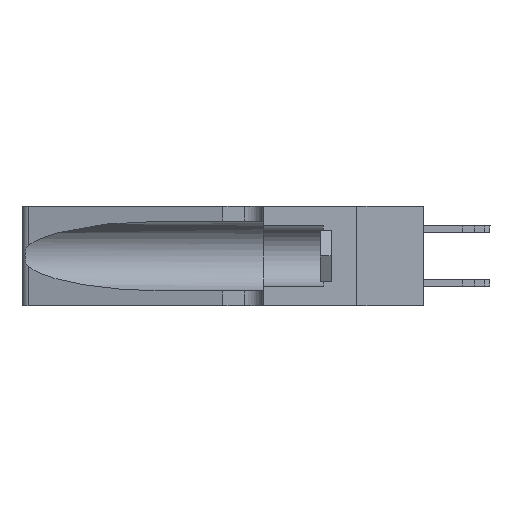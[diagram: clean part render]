
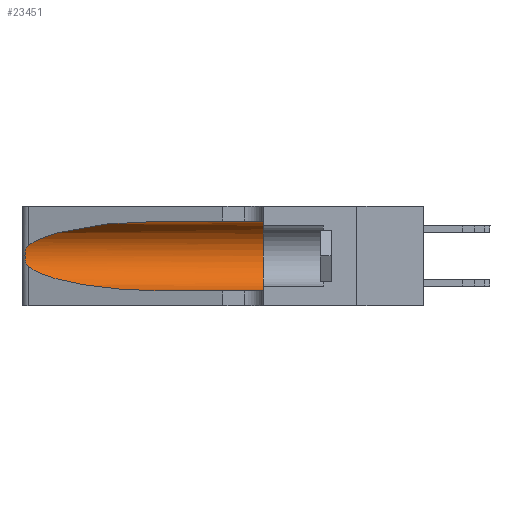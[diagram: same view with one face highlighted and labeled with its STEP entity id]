
A CAD part, left-side view. The second image highlights one B-rep face of the part: STEP entity #23451.
In plain terms, the highlighted cylindrical face has radius 3.308 mm (diameter 6.617 mm), a partial arc.
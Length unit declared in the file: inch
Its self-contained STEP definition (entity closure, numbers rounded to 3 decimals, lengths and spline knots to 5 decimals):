
#1413 = ORIENTED_EDGE ( 'NONE', *, *, #24359, .F. ) ;
#1736 = CARTESIAN_POINT ( 'NONE',  ( 0.26018, 1.23835, 0.19895 ) ) ;
#1756 = CARTESIAN_POINT ( 'NONE',  ( 0.1305, 0.35, 0.31525 ) ) ;
#2377 = CARTESIAN_POINT ( 'NONE',  ( 0.25639, 1.23184, 0.21858 ) ) ;
#2514 = CARTESIAN_POINT ( 'NONE',  ( 0.1305, 0.35, 0.05475 ) ) ;
#2838 =( BOUNDED_CURVE ( )  B_SPLINE_CURVE ( 3, ( #18776, #30843, #30980, #16285 ),
 .UNSPECIFIED., .F., .T. ) 
 B_SPLINE_CURVE_WITH_KNOTS ( ( 4, 4 ),
 ( 3.44316, 4.71239 ),
 .UNSPECIFIED. ) 
 CURVE ( )  GEOMETRIC_REPRESENTATION_ITEM ( )  RATIONAL_B_SPLINE_CURVE ( ( 1., 0.87, 0.87, 1. ) ) 
 REPRESENTATION_ITEM ( '' )  );
#3918 = ORIENTED_EDGE ( 'NONE', *, *, #34182, .T. ) ;
#4420 = CARTESIAN_POINT ( 'NONE',  ( 0.25487, 1.22718, 0.22369 ) ) ;
#5197 = EDGE_CURVE ( 'NONE', #24166, #35041, #21450, .T. ) ;
#5896 = EDGE_CURVE ( 'NONE', #35041, #34052, #2838, .T. ) ;
#6959 = CIRCLE ( 'NONE', #14905, 0.13025 ) ;
#7319 = CARTESIAN_POINT ( 'NONE',  ( 0.25856, 1.23593, 0.16098 ) ) ;
#9379 = DIRECTION ( 'NONE',  ( 0., -1., 0. ) ) ;
#10351 = CARTESIAN_POINT ( 'NONE',  ( 0.25639, 1.23186, 0.15144 ) ) ;
#11080 = CARTESIAN_POINT ( 'NONE',  ( 0.25487, 1.22718, 0.14631 ) ) ;
#13083 = DIRECTION ( 'NONE',  ( 0., -1., 0. ) ) ;
#13491 = CARTESIAN_POINT ( 'NONE',  ( 0.25555, 1.22993, 0.14849 ) ) ;
#14083 = LINE ( 'NONE', #30798, #19252 ) ;
#14431 = ORIENTED_EDGE ( 'NONE', *, *, #5197, .T. ) ;
#14905 = AXIS2_PLACEMENT_3D ( 'NONE', #33902, #27974, #21944 ) ;
#15309 = EDGE_CURVE ( 'NONE', #31560, #19683, #14083, .T. ) ;
#15947 = FACE_OUTER_BOUND ( 'NONE', #31369, .T. ) ;
#16285 = CARTESIAN_POINT ( 'NONE',  ( 0.1305, 0.72297, 0.05475 ) ) ;
#16299 = ORIENTED_EDGE ( 'NONE', *, *, #15309, .F. ) ;
#18776 = CARTESIAN_POINT ( 'NONE',  ( 0.25487, 1.22718, 0.14631 ) ) ;
#19252 = VECTOR ( 'NONE', #13083, 39.37008 ) ;
#19399 = CARTESIAN_POINT ( 'NONE',  ( 0.25854, 1.2359, 0.20912 ) ) ;
#19663 = CARTESIAN_POINT ( 'NONE',  ( 0.26075, 1.23896, 0.19203 ) ) ;
#19683 = VERTEX_POINT ( 'NONE', #1756 ) ;
#20641 = EDGE_CURVE ( 'NONE', #34052, #34509, #30202, .T. ) ;
#21450 = B_SPLINE_CURVE_WITH_KNOTS ( 'NONE', 3,
 ( #31483, #32399, #2377, #31736, #19399, #1736, #19663, #23468, #25331, #7319, #28320, #10351, #13491, #34374 ),
 .UNSPECIFIED., .F., .F.,
 ( 4, 2, 2, 2, 2, 2, 4 ),
 ( 0., 0.00027, 0.00053, 0.00107, 0.0016, 0.00187, 0.00214 ),
 .UNSPECIFIED. ) ;
#21944 = DIRECTION ( 'NONE',  ( 0., 0., 1. ) ) ;
#22070 = CARTESIAN_POINT ( 'NONE',  ( 0.1305, 0.72297, 0.05475 ) ) ;
#22495 = ORIENTED_EDGE ( 'NONE', *, *, #20641, .T. ) ;
#22784 = CARTESIAN_POINT ( 'NONE',  ( 0.1305, 0.72297, 0.31525 ) ) ;
#22894 =( BOUNDED_CURVE ( )  B_SPLINE_CURVE ( 3, ( #33502, #36501, #27957, #4420 ),
 .UNSPECIFIED., .F., .F. ) 
 B_SPLINE_CURVE_WITH_KNOTS ( ( 4, 4 ),
 ( 1.5708, 2.84003 ),
 .UNSPECIFIED. ) 
 CURVE ( )  GEOMETRIC_REPRESENTATION_ITEM ( )  RATIONAL_B_SPLINE_CURVE ( ( 1., 0.87, 0.87, 1. ) ) 
 REPRESENTATION_ITEM ( '' )  );
#22989 = AXIS2_PLACEMENT_3D ( 'NONE', #32690, #38712, #29890 ) ;
#23451 = ADVANCED_FACE ( 'NONE', ( #15947 ), #25823, .F. ) ;
#23468 = CARTESIAN_POINT ( 'NONE',  ( 0.26075, 1.23896, 0.178 ) ) ;
#24166 = VERTEX_POINT ( 'NONE', #26969 ) ;
#24359 = EDGE_CURVE ( 'NONE', #19683, #34509, #6959, .T. ) ;
#25331 = CARTESIAN_POINT ( 'NONE',  ( 0.26017, 1.23833, 0.17102 ) ) ;
#25823 = CYLINDRICAL_SURFACE ( 'NONE', #22989, 0.13025 ) ;
#26300 = CARTESIAN_POINT ( 'NONE',  ( 0.1305, 1.61858, 0.05475 ) ) ;
#26969 = CARTESIAN_POINT ( 'NONE',  ( 0.25487, 1.22718, 0.22369 ) ) ;
#27385 = VECTOR ( 'NONE', #9379, 39.37008 ) ;
#27957 = CARTESIAN_POINT ( 'NONE',  ( 0.2373, 1.15595, 0.28018 ) ) ;
#27974 = DIRECTION ( 'NONE',  ( 0., 1., 0. ) ) ;
#28320 = CARTESIAN_POINT ( 'NONE',  ( 0.25789, 1.23486, 0.15765 ) ) ;
#29890 = DIRECTION ( 'NONE',  ( 0., 0., -1. ) ) ;
#30202 = LINE ( 'NONE', #26300, #27385 ) ;
#30798 = CARTESIAN_POINT ( 'NONE',  ( 0.1305, 1.61858, 0.31525 ) ) ;
#30843 = CARTESIAN_POINT ( 'NONE',  ( 0.2373, 1.15595, 0.08982 ) ) ;
#30980 = CARTESIAN_POINT ( 'NONE',  ( 0.18966, 0.96281, 0.05475 ) ) ;
#31369 = EDGE_LOOP ( 'NONE', ( #3918, #14431, #31398, #22495, #1413, #16299 ) ) ;
#31398 = ORIENTED_EDGE ( 'NONE', *, *, #5896, .T. ) ;
#31483 = CARTESIAN_POINT ( 'NONE',  ( 0.25487, 1.22718, 0.22369 ) ) ;
#31560 = VERTEX_POINT ( 'NONE', #22784 ) ;
#31736 = CARTESIAN_POINT ( 'NONE',  ( 0.25787, 1.23484, 0.2124 ) ) ;
#32399 = CARTESIAN_POINT ( 'NONE',  ( 0.25555, 1.22994, 0.2215 ) ) ;
#32690 = CARTESIAN_POINT ( 'NONE',  ( 0.1305, 1.61858, 0.185 ) ) ;
#33502 = CARTESIAN_POINT ( 'NONE',  ( 0.1305, 0.72297, 0.31525 ) ) ;
#33902 = CARTESIAN_POINT ( 'NONE',  ( 0.1305, 0.35, 0.185 ) ) ;
#34052 = VERTEX_POINT ( 'NONE', #22070 ) ;
#34182 = EDGE_CURVE ( 'NONE', #31560, #24166, #22894, .T. ) ;
#34374 = CARTESIAN_POINT ( 'NONE',  ( 0.25487, 1.22718, 0.14631 ) ) ;
#34509 = VERTEX_POINT ( 'NONE', #2514 ) ;
#35041 = VERTEX_POINT ( 'NONE', #11080 ) ;
#36501 = CARTESIAN_POINT ( 'NONE',  ( 0.18966, 0.96281, 0.31525 ) ) ;
#38712 = DIRECTION ( 'NONE',  ( 0., -1., 0. ) ) ;
